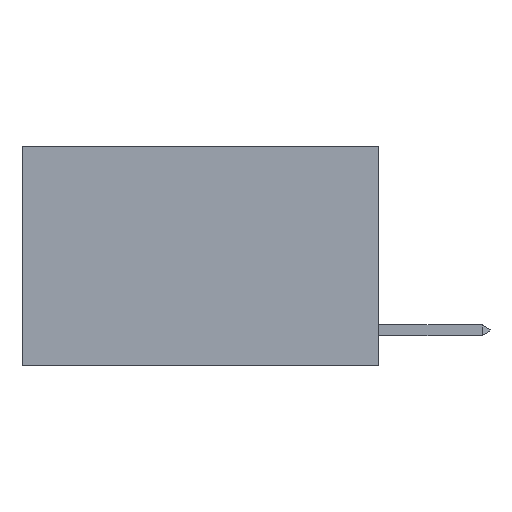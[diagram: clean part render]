
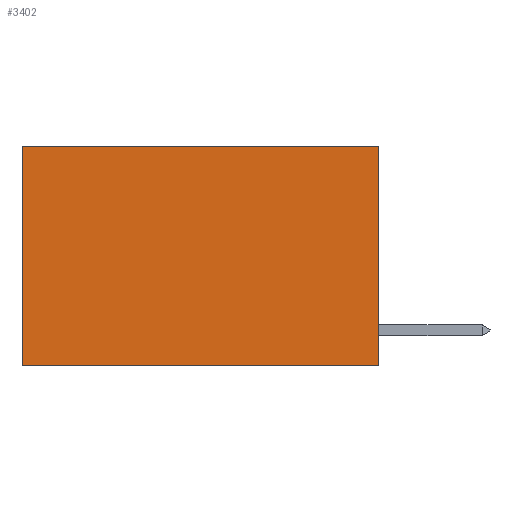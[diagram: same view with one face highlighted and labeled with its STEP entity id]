
A CAD part, left-side view. The second image highlights one B-rep face of the part: STEP entity #3402.
In plain terms, the highlighted planar face has unit normal (-1, 0, 0).
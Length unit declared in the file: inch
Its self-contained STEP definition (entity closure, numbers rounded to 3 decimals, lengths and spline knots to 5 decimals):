
#12 = ORIENTED_EDGE ( 'NONE', *, *, #2531, .T. ) ;
#89 = CARTESIAN_POINT ( 'NONE',  ( 0.2625, 0., 0. ) ) ;
#126 = VECTOR ( 'NONE', #6114, 39.37008 ) ;
#1073 = LINE ( 'NONE', #6005, #5332 ) ;
#1103 = DIRECTION ( 'NONE',  ( 0., 0., -1. ) ) ;
#1759 = DIRECTION ( 'NONE',  ( 1., 0., 0. ) ) ;
#1948 = DIRECTION ( 'NONE',  ( 0., 1., 0. ) ) ;
#1982 = ORIENTED_EDGE ( 'NONE', *, *, #6708, .F. ) ;
#2531 = EDGE_CURVE ( 'NONE', #5328, #8526, #7987, .T. ) ;
#2700 = CARTESIAN_POINT ( 'NONE',  ( 0.2625, 0., 0. ) ) ;
#2831 = EDGE_CURVE ( 'NONE', #8526, #2920, #4302, .T. ) ;
#2920 = VERTEX_POINT ( 'NONE', #7132 ) ;
#2941 = EDGE_CURVE ( 'NONE', #8312, #2920, #1073, .T. ) ;
#2984 = ORIENTED_EDGE ( 'NONE', *, *, #2941, .F. ) ;
#3402 = ADVANCED_FACE ( 'NONE', ( #8089 ), #5262, .F. ) ;
#3531 = LINE ( 'NONE', #89, #5122 ) ;
#3650 = CARTESIAN_POINT ( 'NONE',  ( 0.2625, 0., -0.37 ) ) ;
#3669 = CARTESIAN_POINT ( 'NONE',  ( 0.2625, 0.6, 0. ) ) ;
#4302 = LINE ( 'NONE', #3669, #5783 ) ;
#4396 = EDGE_LOOP ( 'NONE', ( #5105, #2984, #1982, #12 ) ) ;
#5105 = ORIENTED_EDGE ( 'NONE', *, *, #2831, .T. ) ;
#5122 = VECTOR ( 'NONE', #7566, 39.37008 ) ;
#5262 = PLANE ( 'NONE',  #6359 ) ;
#5328 = VERTEX_POINT ( 'NONE', #6443 ) ;
#5332 = VECTOR ( 'NONE', #1948, 39.37008 ) ;
#5783 = VECTOR ( 'NONE', #7852, 39.37008 ) ;
#6005 = CARTESIAN_POINT ( 'NONE',  ( 0.2625, 0., -0.37 ) ) ;
#6114 = DIRECTION ( 'NONE',  ( 0., 1., 0. ) ) ;
#6359 = AXIS2_PLACEMENT_3D ( 'NONE', #7927, #1759, #1103 ) ;
#6443 = CARTESIAN_POINT ( 'NONE',  ( 0.2625, 0., 0. ) ) ;
#6708 = EDGE_CURVE ( 'NONE', #5328, #8312, #3531, .T. ) ;
#7132 = CARTESIAN_POINT ( 'NONE',  ( 0.2625, 0.6, -0.37 ) ) ;
#7566 = DIRECTION ( 'NONE',  ( 0., 0., -1. ) ) ;
#7852 = DIRECTION ( 'NONE',  ( 0., 0., -1. ) ) ;
#7927 = CARTESIAN_POINT ( 'NONE',  ( 0.2625, 0., 0. ) ) ;
#7987 = LINE ( 'NONE', #2700, #126 ) ;
#8089 = FACE_OUTER_BOUND ( 'NONE', #4396, .T. ) ;
#8312 = VERTEX_POINT ( 'NONE', #3650 ) ;
#8526 = VERTEX_POINT ( 'NONE', #8630 ) ;
#8630 = CARTESIAN_POINT ( 'NONE',  ( 0.2625, 0.6, 0. ) ) ;
